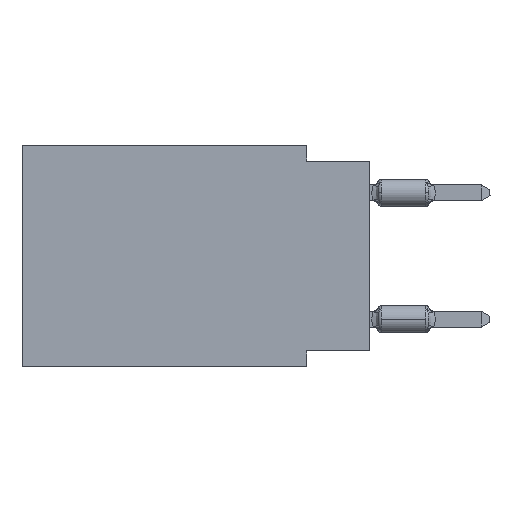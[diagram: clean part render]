
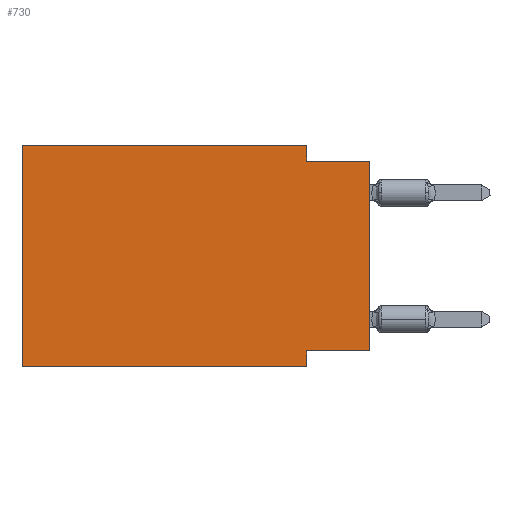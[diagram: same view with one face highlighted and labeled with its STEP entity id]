
A CAD part, left-side view. The second image highlights one B-rep face of the part: STEP entity #730.
In plain terms, the highlighted planar face has unit normal (-1, 0, 0).
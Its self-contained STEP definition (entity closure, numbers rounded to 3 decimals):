
#199 = CARTESIAN_POINT ( 'NONE',  ( 0., 13.97, 0. ) ) ;
#523 = EDGE_CURVE ( 'NONE', #1248, #11758, #25816, .T. ) ;
#730 = ADVANCED_FACE ( 'NONE', ( #18276 ), #4592, .F. ) ;
#1248 = VERTEX_POINT ( 'NONE', #43834 ) ;
#1718 = ORIENTED_EDGE ( 'NONE', *, *, #523, .F. ) ;
#1757 = CARTESIAN_POINT ( 'NONE',  ( 0., 2.54, -8.255 ) ) ;
#2280 = DIRECTION ( 'NONE',  ( 0., -1., 0. ) ) ;
#2518 = VECTOR ( 'NONE', #21548, 1000. ) ;
#4592 = PLANE ( 'NONE',  #17611 ) ;
#4868 = EDGE_CURVE ( 'NONE', #23393, #25922, #25080, .T. ) ;
#5022 = ORIENTED_EDGE ( 'NONE', *, *, #34431, .F. ) ;
#5488 = DIRECTION ( 'NONE',  ( 0., 0., -1. ) ) ;
#5551 = VERTEX_POINT ( 'NONE', #30605 ) ;
#6075 = CARTESIAN_POINT ( 'NONE',  ( 0., 13.97, -8.89 ) ) ;
#6778 = VECTOR ( 'NONE', #2280, 1000. ) ;
#7099 = EDGE_CURVE ( 'NONE', #11758, #40361, #21834, .T. ) ;
#7286 = ORIENTED_EDGE ( 'NONE', *, *, #35096, .F. ) ;
#7483 = VECTOR ( 'NONE', #39435, 1000. ) ;
#8213 = LINE ( 'NONE', #15845, #7483 ) ;
#8428 = EDGE_CURVE ( 'NONE', #23393, #24626, #8213, .T. ) ;
#8750 = CARTESIAN_POINT ( 'NONE',  ( 0., 13.97, 0. ) ) ;
#8876 = EDGE_CURVE ( 'NONE', #1248, #34464, #36839, .T. ) ;
#11758 = VERTEX_POINT ( 'NONE', #199 ) ;
#11761 = EDGE_CURVE ( 'NONE', #25922, #34464, #37467, .T. ) ;
#12727 = ORIENTED_EDGE ( 'NONE', *, *, #11761, .F. ) ;
#15845 = CARTESIAN_POINT ( 'NONE',  ( 0., 0., 0. ) ) ;
#16475 = LINE ( 'NONE', #43010, #29075 ) ;
#16814 = VECTOR ( 'NONE', #22063, 1000. ) ;
#17611 = AXIS2_PLACEMENT_3D ( 'NONE', #25703, #35801, #18732 ) ;
#18276 = FACE_OUTER_BOUND ( 'NONE', #29620, .T. ) ;
#18732 = DIRECTION ( 'NONE',  ( 0., 0., -1. ) ) ;
#20178 = DIRECTION ( 'NONE',  ( 0., 0., -1. ) ) ;
#21548 = DIRECTION ( 'NONE',  ( 0., -1., 0. ) ) ;
#21834 = LINE ( 'NONE', #31278, #16814 ) ;
#22063 = DIRECTION ( 'NONE',  ( 0., -1., 0. ) ) ;
#22296 = CARTESIAN_POINT ( 'NONE',  ( 0., 0., -8.255 ) ) ;
#22439 = DIRECTION ( 'NONE',  ( 0., 0., 1. ) ) ;
#23393 = VERTEX_POINT ( 'NONE', #22296 ) ;
#24626 = VERTEX_POINT ( 'NONE', #26576 ) ;
#25080 = LINE ( 'NONE', #36301, #35400 ) ;
#25703 = CARTESIAN_POINT ( 'NONE',  ( 0., 13.97, 0. ) ) ;
#25816 = LINE ( 'NONE', #8750, #42453 ) ;
#25922 = VERTEX_POINT ( 'NONE', #1757 ) ;
#26576 = CARTESIAN_POINT ( 'NONE',  ( 0., 0., -0.635 ) ) ;
#28894 = ORIENTED_EDGE ( 'NONE', *, *, #4868, .F. ) ;
#29075 = VECTOR ( 'NONE', #5488, 1000. ) ;
#29620 = EDGE_LOOP ( 'NONE', ( #41487, #7286, #5022, #39185, #1718, #35272, #12727, #28894 ) ) ;
#30425 = CARTESIAN_POINT ( 'NONE',  ( 0., 2.54, 0. ) ) ;
#30605 = CARTESIAN_POINT ( 'NONE',  ( 0., 2.54, -0.635 ) ) ;
#31278 = CARTESIAN_POINT ( 'NONE',  ( 0., 13.97, 0. ) ) ;
#34431 = EDGE_CURVE ( 'NONE', #40361, #5551, #16475, .T. ) ;
#34464 = VERTEX_POINT ( 'NONE', #36251 ) ;
#35096 = EDGE_CURVE ( 'NONE', #5551, #24626, #41555, .T. ) ;
#35272 = ORIENTED_EDGE ( 'NONE', *, *, #8876, .T. ) ;
#35400 = VECTOR ( 'NONE', #35403, 1000. ) ;
#35403 = DIRECTION ( 'NONE',  ( 0., 1., 0. ) ) ;
#35801 = DIRECTION ( 'NONE',  ( 1., 0., 0. ) ) ;
#36251 = CARTESIAN_POINT ( 'NONE',  ( 0., 2.54, -8.89 ) ) ;
#36301 = CARTESIAN_POINT ( 'NONE',  ( 0., 0., -8.255 ) ) ;
#36839 = LINE ( 'NONE', #6075, #6778 ) ;
#37254 = CARTESIAN_POINT ( 'NONE',  ( 0., 2.54, -8.89 ) ) ;
#37467 = LINE ( 'NONE', #37254, #39499 ) ;
#38175 = CARTESIAN_POINT ( 'NONE',  ( 0., 0., -0.635 ) ) ;
#39185 = ORIENTED_EDGE ( 'NONE', *, *, #7099, .F. ) ;
#39435 = DIRECTION ( 'NONE',  ( 0., 0., 1. ) ) ;
#39499 = VECTOR ( 'NONE', #20178, 1000. ) ;
#40361 = VERTEX_POINT ( 'NONE', #30425 ) ;
#41487 = ORIENTED_EDGE ( 'NONE', *, *, #8428, .T. ) ;
#41555 = LINE ( 'NONE', #38175, #2518 ) ;
#42453 = VECTOR ( 'NONE', #22439, 1000. ) ;
#43010 = CARTESIAN_POINT ( 'NONE',  ( 0., 2.54, 0. ) ) ;
#43834 = CARTESIAN_POINT ( 'NONE',  ( 0., 13.97, -8.89 ) ) ;
